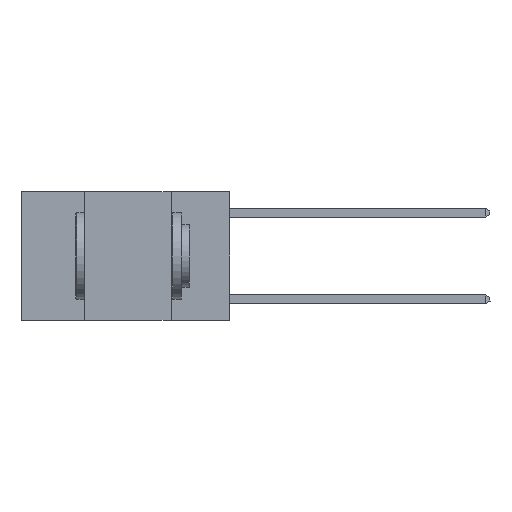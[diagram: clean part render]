
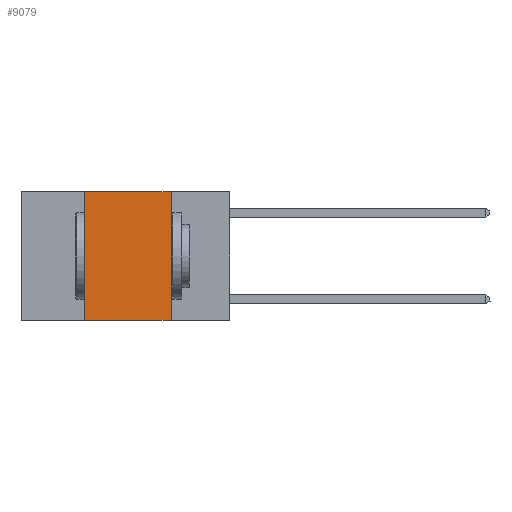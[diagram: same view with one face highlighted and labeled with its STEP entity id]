
A CAD part, left-side view. The second image highlights one B-rep face of the part: STEP entity #9079.
In plain terms, the highlighted planar face has unit normal (-1, 0, 0).
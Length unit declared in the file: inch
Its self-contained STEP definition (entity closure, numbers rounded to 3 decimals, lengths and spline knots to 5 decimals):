
#540 = DIRECTION ( 'NONE',  ( 0., 0., 1. ) ) ;
#1066 = VERTEX_POINT ( 'NONE', #17540 ) ;
#1650 = VECTOR ( 'NONE', #15741, 39.37008 ) ;
#2229 = DIRECTION ( 'NONE',  ( 1., 0., 0. ) ) ;
#2885 = LINE ( 'NONE', #9256, #10694 ) ;
#3204 = EDGE_CURVE ( 'NONE', #1066, #16795, #15443, .T. ) ;
#3241 = CARTESIAN_POINT ( 'NONE',  ( 0., 0.42, -0.37 ) ) ;
#5700 = FACE_OUTER_BOUND ( 'NONE', #15807, .T. ) ;
#6387 = CARTESIAN_POINT ( 'NONE',  ( 0., 0.17, 0. ) ) ;
#6870 = CARTESIAN_POINT ( 'NONE',  ( 0., 0.17, -0.37 ) ) ;
#7724 = EDGE_CURVE ( 'NONE', #16795, #7952, #9915, .T. ) ;
#7952 = VERTEX_POINT ( 'NONE', #6870 ) ;
#8044 = DIRECTION ( 'NONE',  ( 0., -1., 0. ) ) ;
#8988 = LINE ( 'NONE', #19011, #16717 ) ;
#9079 = ADVANCED_FACE ( 'NONE', ( #5700 ), #19072, .F. ) ;
#9256 = CARTESIAN_POINT ( 'NONE',  ( 0., 0.6, -0.37 ) ) ;
#9915 = LINE ( 'NONE', #6387, #1650 ) ;
#10694 = VECTOR ( 'NONE', #10838, 39.37008 ) ;
#10838 = DIRECTION ( 'NONE',  ( 0., -1., 0. ) ) ;
#10914 = VERTEX_POINT ( 'NONE', #3241 ) ;
#11270 = EDGE_CURVE ( 'NONE', #10914, #7952, #2885, .T. ) ;
#11326 = VECTOR ( 'NONE', #8044, 39.37008 ) ;
#11588 = CARTESIAN_POINT ( 'NONE',  ( 0., 0.6, 0. ) ) ;
#12345 = ORIENTED_EDGE ( 'NONE', *, *, #7724, .F. ) ;
#13118 = DIRECTION ( 'NONE',  ( 0., 0., -1. ) ) ;
#15443 = LINE ( 'NONE', #15847, #11326 ) ;
#15741 = DIRECTION ( 'NONE',  ( 0., 0., -1. ) ) ;
#15807 = EDGE_LOOP ( 'NONE', ( #12345, #18367, #19033, #16491 ) ) ;
#15847 = CARTESIAN_POINT ( 'NONE',  ( 0., 0.6, 0. ) ) ;
#16491 = ORIENTED_EDGE ( 'NONE', *, *, #11270, .T. ) ;
#16717 = VECTOR ( 'NONE', #540, 39.37008 ) ;
#16795 = VERTEX_POINT ( 'NONE', #18686 ) ;
#17422 = EDGE_CURVE ( 'NONE', #10914, #1066, #8988, .T. ) ;
#17540 = CARTESIAN_POINT ( 'NONE',  ( 0., 0.42, 0. ) ) ;
#17706 = AXIS2_PLACEMENT_3D ( 'NONE', #11588, #2229, #13118 ) ;
#18367 = ORIENTED_EDGE ( 'NONE', *, *, #3204, .F. ) ;
#18686 = CARTESIAN_POINT ( 'NONE',  ( 0., 0.17, 0. ) ) ;
#19011 = CARTESIAN_POINT ( 'NONE',  ( 0., 0.42, 0. ) ) ;
#19033 = ORIENTED_EDGE ( 'NONE', *, *, #17422, .F. ) ;
#19072 = PLANE ( 'NONE',  #17706 ) ;
